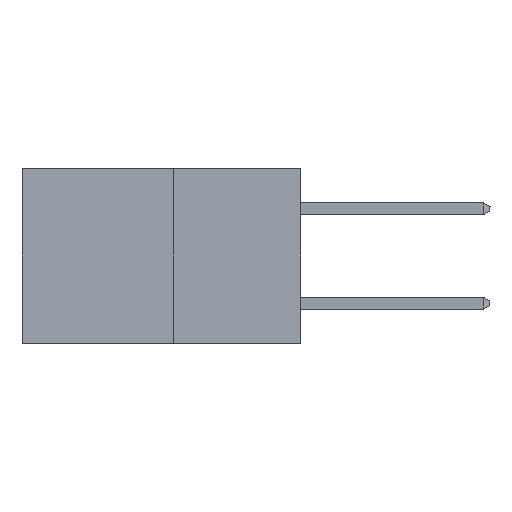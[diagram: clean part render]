
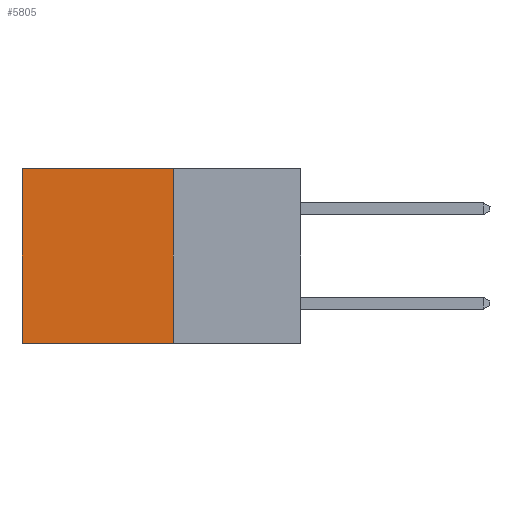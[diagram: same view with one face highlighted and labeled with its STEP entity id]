
A CAD part, left-side view. The second image highlights one B-rep face of the part: STEP entity #5805.
In plain terms, the highlighted planar face has unit normal (-1, 0, 0).
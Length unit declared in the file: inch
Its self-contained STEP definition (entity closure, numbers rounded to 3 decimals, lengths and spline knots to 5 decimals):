
#387 = VERTEX_POINT ( 'NONE', #1072 ) ;
#789 = CARTESIAN_POINT ( 'NONE',  ( 0.277, 0.27, -0.37 ) ) ;
#853 = LINE ( 'NONE', #789, #8908 ) ;
#1072 = CARTESIAN_POINT ( 'NONE',  ( 0.277, 0.59, 0. ) ) ;
#1169 = CARTESIAN_POINT ( 'NONE',  ( 0.277, 0.59, -0.37 ) ) ;
#1557 = EDGE_LOOP ( 'NONE', ( #11446, #6216, #6541, #9268 ) ) ;
#2433 = VECTOR ( 'NONE', #12238, 39.37008 ) ;
#2529 = VECTOR ( 'NONE', #4788, 39.37008 ) ;
#2611 = CARTESIAN_POINT ( 'NONE',  ( 0.277, 0.27, -0.37 ) ) ;
#2972 = VERTEX_POINT ( 'NONE', #1169 ) ;
#3613 = FACE_OUTER_BOUND ( 'NONE', #1557, .T. ) ;
#4643 = VECTOR ( 'NONE', #11628, 39.37008 ) ;
#4788 = DIRECTION ( 'NONE',  ( 0., 0., -1. ) ) ;
#4839 = EDGE_CURVE ( 'NONE', #10706, #387, #10486, .T. ) ;
#4882 = EDGE_CURVE ( 'NONE', #387, #2972, #7673, .T. ) ;
#5001 = DIRECTION ( 'NONE',  ( 0., 0., -1. ) ) ;
#5019 = DIRECTION ( 'NONE',  ( 1., 0., 0. ) ) ;
#5030 = CARTESIAN_POINT ( 'NONE',  ( 0.277, 0.27, -0.37 ) ) ;
#5183 = PLANE ( 'NONE',  #12755 ) ;
#5190 = VERTEX_POINT ( 'NONE', #9205 ) ;
#5389 = LINE ( 'NONE', #2611, #2529 ) ;
#5805 = ADVANCED_FACE ( 'NONE', ( #3613 ), #5183, .F. ) ;
#6216 = ORIENTED_EDGE ( 'NONE', *, *, #6456, .F. ) ;
#6456 = EDGE_CURVE ( 'NONE', #5190, #2972, #853, .T. ) ;
#6541 = ORIENTED_EDGE ( 'NONE', *, *, #11789, .F. ) ;
#7187 = DIRECTION ( 'NONE',  ( 0., 1., 0. ) ) ;
#7673 = LINE ( 'NONE', #11645, #4643 ) ;
#8908 = VECTOR ( 'NONE', #7187, 39.37008 ) ;
#9205 = CARTESIAN_POINT ( 'NONE',  ( 0.277, 0.27, -0.37 ) ) ;
#9268 = ORIENTED_EDGE ( 'NONE', *, *, #4839, .T. ) ;
#10486 = LINE ( 'NONE', #12192, #2433 ) ;
#10706 = VERTEX_POINT ( 'NONE', #12489 ) ;
#11446 = ORIENTED_EDGE ( 'NONE', *, *, #4882, .T. ) ;
#11628 = DIRECTION ( 'NONE',  ( 0., 0., -1. ) ) ;
#11645 = CARTESIAN_POINT ( 'NONE',  ( 0.277, 0.59, -0.37 ) ) ;
#11789 = EDGE_CURVE ( 'NONE', #10706, #5190, #5389, .T. ) ;
#12192 = CARTESIAN_POINT ( 'NONE',  ( 0.277, 0.27, 0. ) ) ;
#12238 = DIRECTION ( 'NONE',  ( 0., 1., 0. ) ) ;
#12489 = CARTESIAN_POINT ( 'NONE',  ( 0.277, 0.27, 0. ) ) ;
#12755 = AXIS2_PLACEMENT_3D ( 'NONE', #5030, #5019, #5001 ) ;
